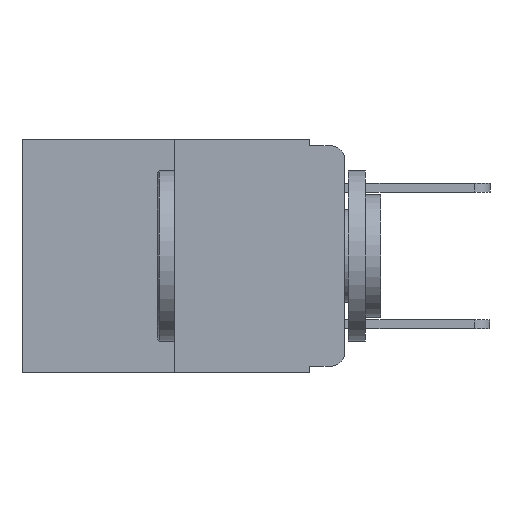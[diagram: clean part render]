
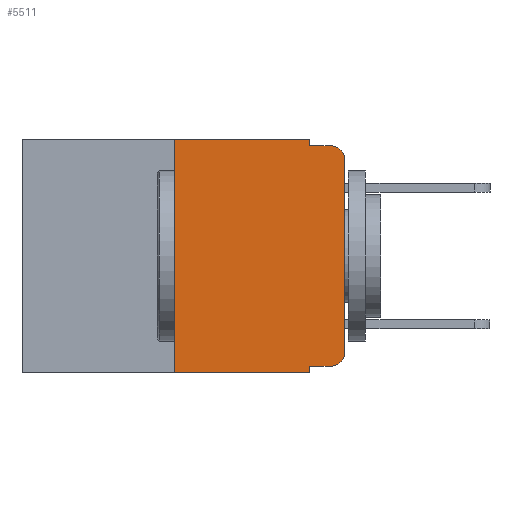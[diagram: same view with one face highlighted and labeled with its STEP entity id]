
A CAD part, left-side view. The second image highlights one B-rep face of the part: STEP entity #5511.
In plain terms, the highlighted planar face has unit normal (-1, 0, 0).
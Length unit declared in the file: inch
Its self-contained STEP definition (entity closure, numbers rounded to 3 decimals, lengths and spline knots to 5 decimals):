
#66 = EDGE_CURVE ( 'NONE', #24010, #942, #11061, .T. ) ;
#281 = PLANE ( 'NONE',  #398 ) ;
#398 = AXIS2_PLACEMENT_3D ( 'NONE', #13493, #15352, #4148 ) ;
#942 = VERTEX_POINT ( 'NONE', #9926 ) ;
#994 = DIRECTION ( 'NONE',  ( 0., 0., 1. ) ) ;
#1060 = CARTESIAN_POINT ( 'NONE',  ( 0., 0.051, -0.333 ) ) ;
#1225 = VECTOR ( 'NONE', #13761, 39.37008 ) ;
#2005 = CARTESIAN_POINT ( 'NONE',  ( 0., 0., -0.313 ) ) ;
#2213 = LINE ( 'NONE', #20499, #21432 ) ;
#2466 = ORIENTED_EDGE ( 'NONE', *, *, #14903, .T. ) ;
#2582 = EDGE_CURVE ( 'NONE', #17361, #6535, #15536, .T. ) ;
#2627 = DIRECTION ( 'NONE',  ( -1., 0., 0. ) ) ;
#2659 = EDGE_CURVE ( 'NONE', #9900, #942, #13789, .T. ) ;
#2867 = CARTESIAN_POINT ( 'NONE',  ( 0., 0.051, 0. ) ) ;
#3216 = VERTEX_POINT ( 'NONE', #23188 ) ;
#3265 = LINE ( 'NONE', #7257, #12089 ) ;
#3326 = LINE ( 'NONE', #21463, #12733 ) ;
#3668 = ORIENTED_EDGE ( 'NONE', *, *, #8699, .T. ) ;
#4148 = DIRECTION ( 'NONE',  ( 0., 0., -1. ) ) ;
#4912 = CARTESIAN_POINT ( 'NONE',  ( 0., 0., -0.03 ) ) ;
#5189 = VECTOR ( 'NONE', #15978, 39.37008 ) ;
#5511 = ADVANCED_FACE ( 'NONE', ( #6435 ), #281, .F. ) ;
#6015 = VECTOR ( 'NONE', #24008, 39.37008 ) ;
#6183 = VECTOR ( 'NONE', #19857, 39.37008 ) ;
#6435 = FACE_OUTER_BOUND ( 'NONE', #15191, .T. ) ;
#6535 = VERTEX_POINT ( 'NONE', #7493 ) ;
#6952 = EDGE_CURVE ( 'NONE', #3216, #7218, #13394, .T. ) ;
#6969 = CARTESIAN_POINT ( 'NONE',  ( 0., 0.25, 0. ) ) ;
#7218 = VERTEX_POINT ( 'NONE', #13058 ) ;
#7257 = CARTESIAN_POINT ( 'NONE',  ( 0., 0.051, 0. ) ) ;
#7493 = CARTESIAN_POINT ( 'NONE',  ( 0., 0.051, 0. ) ) ;
#8699 = EDGE_CURVE ( 'NONE', #23115, #12009, #20249, .T. ) ;
#8793 = CARTESIAN_POINT ( 'NONE',  ( 0., 0.25, -0.343 ) ) ;
#8935 = LINE ( 'NONE', #1060, #18184 ) ;
#9369 = EDGE_CURVE ( 'NONE', #12389, #7218, #20504, .T. ) ;
#9477 = EDGE_CURVE ( 'NONE', #12389, #17361, #3326, .T. ) ;
#9543 = ORIENTED_EDGE ( 'NONE', *, *, #2659, .T. ) ;
#9572 = ORIENTED_EDGE ( 'NONE', *, *, #9369, .T. ) ;
#9900 = VERTEX_POINT ( 'NONE', #4912 ) ;
#9926 = CARTESIAN_POINT ( 'NONE',  ( 0., 0.02, -0.01 ) ) ;
#10480 = DIRECTION ( 'NONE',  ( 0., 0., -1. ) ) ;
#10731 = ORIENTED_EDGE ( 'NONE', *, *, #66, .F. ) ;
#10756 = ORIENTED_EDGE ( 'NONE', *, *, #6952, .F. ) ;
#11061 = LINE ( 'NONE', #21364, #6015 ) ;
#11161 = DIRECTION ( 'NONE',  ( -1., 0., 0. ) ) ;
#11243 = CARTESIAN_POINT ( 'NONE',  ( 0., 0.02, -0.03 ) ) ;
#11608 = ORIENTED_EDGE ( 'NONE', *, *, #2582, .F. ) ;
#12009 = VERTEX_POINT ( 'NONE', #2005 ) ;
#12089 = VECTOR ( 'NONE', #18384, 39.37008 ) ;
#12389 = VERTEX_POINT ( 'NONE', #8793 ) ;
#12615 = CARTESIAN_POINT ( 'NONE',  ( 0., 0.051, -0.01 ) ) ;
#12733 = VECTOR ( 'NONE', #994, 39.37008 ) ;
#12759 = EDGE_CURVE ( 'NONE', #12009, #9900, #2213, .T. ) ;
#13058 = CARTESIAN_POINT ( 'NONE',  ( 0., 0.051, -0.343 ) ) ;
#13394 = LINE ( 'NONE', #2867, #5189 ) ;
#13493 = CARTESIAN_POINT ( 'NONE',  ( 0., 0.473, 0. ) ) ;
#13761 = DIRECTION ( 'NONE',  ( 0., -1., 0. ) ) ;
#13789 = CIRCLE ( 'NONE', #13936, 0.02 ) ;
#13844 = CARTESIAN_POINT ( 'NONE',  ( 0., 0.473, -0.343 ) ) ;
#13870 = CARTESIAN_POINT ( 'NONE',  ( 0., 0.02, -0.313 ) ) ;
#13936 = AXIS2_PLACEMENT_3D ( 'NONE', #11243, #11161, #10480 ) ;
#14213 = DIRECTION ( 'NONE',  ( 0., -1., 0. ) ) ;
#14903 = EDGE_CURVE ( 'NONE', #3216, #23115, #8935, .T. ) ;
#15191 = EDGE_LOOP ( 'NONE', ( #18217, #9543, #10731, #23970, #11608, #21966, #9572, #10756, #2466, #3668 ) ) ;
#15352 = DIRECTION ( 'NONE',  ( 1., 0., 0. ) ) ;
#15536 = LINE ( 'NONE', #19747, #6183 ) ;
#15736 = DIRECTION ( 'NONE',  ( 0., 0., -1. ) ) ;
#15978 = DIRECTION ( 'NONE',  ( 0., 0., -1. ) ) ;
#17361 = VERTEX_POINT ( 'NONE', #6969 ) ;
#18156 = EDGE_CURVE ( 'NONE', #6535, #24010, #3265, .T. ) ;
#18184 = VECTOR ( 'NONE', #14213, 39.37008 ) ;
#18217 = ORIENTED_EDGE ( 'NONE', *, *, #12759, .T. ) ;
#18384 = DIRECTION ( 'NONE',  ( 0., 0., -1. ) ) ;
#18741 = DIRECTION ( 'NONE',  ( 0., 0., 1. ) ) ;
#19257 = CARTESIAN_POINT ( 'NONE',  ( 0., 0.02, -0.333 ) ) ;
#19747 = CARTESIAN_POINT ( 'NONE',  ( 0., 0.473, 0. ) ) ;
#19857 = DIRECTION ( 'NONE',  ( 0., -1., 0. ) ) ;
#20084 = AXIS2_PLACEMENT_3D ( 'NONE', #13870, #2627, #15736 ) ;
#20249 = CIRCLE ( 'NONE', #20084, 0.02 ) ;
#20499 = CARTESIAN_POINT ( 'NONE',  ( 0., 0., 0. ) ) ;
#20504 = LINE ( 'NONE', #13844, #1225 ) ;
#21364 = CARTESIAN_POINT ( 'NONE',  ( 0., 0.051, -0.01 ) ) ;
#21432 = VECTOR ( 'NONE', #18741, 39.37008 ) ;
#21463 = CARTESIAN_POINT ( 'NONE',  ( 0., 0.25, 0. ) ) ;
#21966 = ORIENTED_EDGE ( 'NONE', *, *, #9477, .F. ) ;
#23115 = VERTEX_POINT ( 'NONE', #19257 ) ;
#23188 = CARTESIAN_POINT ( 'NONE',  ( 0., 0.051, -0.333 ) ) ;
#23970 = ORIENTED_EDGE ( 'NONE', *, *, #18156, .F. ) ;
#24008 = DIRECTION ( 'NONE',  ( 0., -1., 0. ) ) ;
#24010 = VERTEX_POINT ( 'NONE', #12615 ) ;
